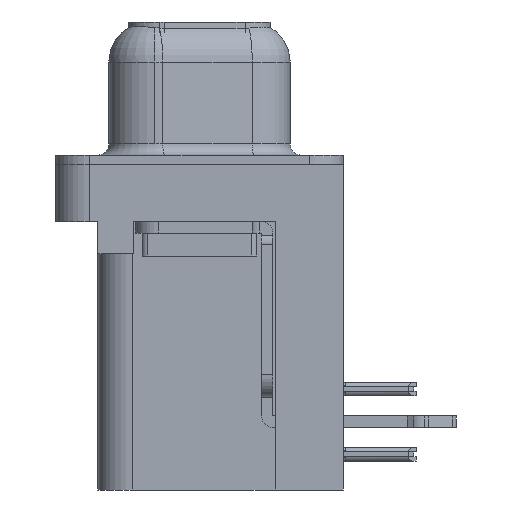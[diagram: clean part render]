
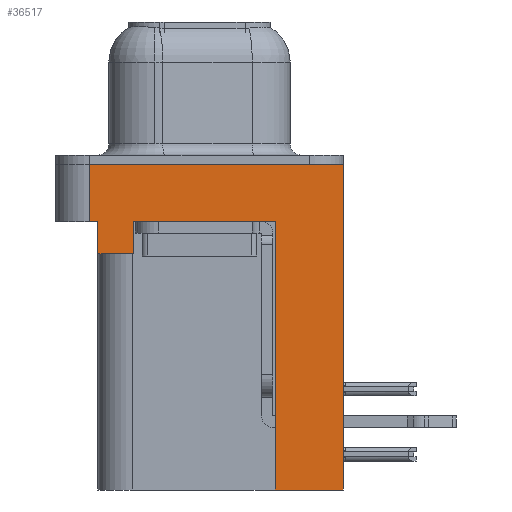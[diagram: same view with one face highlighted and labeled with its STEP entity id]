
A CAD part, left-side view. The second image highlights one B-rep face of the part: STEP entity #36517.
In plain terms, the highlighted planar face has unit normal (-1, 0, 0).
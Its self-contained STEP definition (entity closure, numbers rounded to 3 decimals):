
#898 = DIRECTION ( 'NONE',  ( 0., 0., 1. ) ) ;
#1090 = VERTEX_POINT ( 'NONE', #3404 ) ;
#1162 = CARTESIAN_POINT ( 'NONE',  ( -2.91, 4.425, -2.5 ) ) ;
#2008 = ORIENTED_EDGE ( 'NONE', *, *, #3464, .F. ) ;
#2231 = DIRECTION ( 'NONE',  ( 0., 0., 1. ) ) ;
#2483 = LINE ( 'NONE', #10907, #5870 ) ;
#2527 = LINE ( 'NONE', #36993, #9130 ) ;
#3404 = CARTESIAN_POINT ( 'NONE',  ( -2.91, 4.775, -2.5 ) ) ;
#3464 = EDGE_CURVE ( 'NONE', #19878, #36269, #32067, .T. ) ;
#3587 = EDGE_LOOP ( 'NONE', ( #21074, #10471, #36669, #2008, #30302, #30463, #7401, #21147, #18138, #16201 ) ) ;
#3831 = AXIS2_PLACEMENT_3D ( 'NONE', #22503, #31313, #22687 ) ;
#4296 = EDGE_CURVE ( 'NONE', #1090, #36269, #2483, .T. ) ;
#4725 = LINE ( 'NONE', #10325, #6141 ) ;
#5227 = LINE ( 'NONE', #19285, #10044 ) ;
#5805 = LINE ( 'NONE', #23047, #31759 ) ;
#5870 = VECTOR ( 'NONE', #33771, 1000. ) ;
#6141 = VECTOR ( 'NONE', #13321, 1000. ) ;
#6262 = CARTESIAN_POINT ( 'NONE',  ( -2.91, -6.275, -14.2 ) ) ;
#6846 = VERTEX_POINT ( 'NONE', #6262 ) ;
#7401 = ORIENTED_EDGE ( 'NONE', *, *, #11148, .T. ) ;
#8480 = VERTEX_POINT ( 'NONE', #26962 ) ;
#9016 = DIRECTION ( 'NONE',  ( 0., 0., 1. ) ) ;
#9044 = CARTESIAN_POINT ( 'NONE',  ( -2.91, -3.295, -14.2 ) ) ;
#9060 = DIRECTION ( 'NONE',  ( 0., 1., 0. ) ) ;
#9130 = VECTOR ( 'NONE', #9060, 1000. ) ;
#9145 = CARTESIAN_POINT ( 'NONE',  ( -2.91, 2.895, -3.9 ) ) ;
#9480 = EDGE_CURVE ( 'NONE', #27949, #31424, #14286, .T. ) ;
#9493 = EDGE_CURVE ( 'NONE', #15021, #8480, #26099, .T. ) ;
#9781 = EDGE_CURVE ( 'NONE', #6846, #8480, #5227, .T. ) ;
#10044 = VECTOR ( 'NONE', #2231, 1000. ) ;
#10325 = CARTESIAN_POINT ( 'NONE',  ( -2.91, -6.275, -2.5 ) ) ;
#10471 = ORIENTED_EDGE ( 'NONE', *, *, #26004, .F. ) ;
#10907 = CARTESIAN_POINT ( 'NONE',  ( -2.91, -6.275, -2.5 ) ) ;
#10985 = CARTESIAN_POINT ( 'NONE',  ( -2.91, -3.295, -14.2 ) ) ;
#11148 = EDGE_CURVE ( 'NONE', #25898, #31424, #4725, .T. ) ;
#12255 = CARTESIAN_POINT ( 'NONE',  ( -2.91, 2.895, -3.9 ) ) ;
#12529 = EDGE_CURVE ( 'NONE', #6846, #27949, #36653, .T. ) ;
#12693 = CARTESIAN_POINT ( 'NONE',  ( -2.91, -3.295, -2.5 ) ) ;
#13321 = DIRECTION ( 'NONE',  ( 0., -1., 0. ) ) ;
#14056 = EDGE_CURVE ( 'NONE', #22194, #19878, #2527, .T. ) ;
#14103 = DIRECTION ( 'NONE',  ( 0., 0., 1. ) ) ;
#14286 = LINE ( 'NONE', #9044, #18883 ) ;
#15021 = VERTEX_POINT ( 'NONE', #17429 ) ;
#16201 = ORIENTED_EDGE ( 'NONE', *, *, #9781, .T. ) ;
#16905 = FACE_OUTER_BOUND ( 'NONE', #3587, .T. ) ;
#17429 = CARTESIAN_POINT ( 'NONE',  ( -2.91, 4.775, 0. ) ) ;
#17481 = CARTESIAN_POINT ( 'NONE',  ( -2.91, 4.425, -3.9 ) ) ;
#18138 = ORIENTED_EDGE ( 'NONE', *, *, #12529, .F. ) ;
#18387 = EDGE_CURVE ( 'NONE', #22194, #25898, #29031, .T. ) ;
#18883 = VECTOR ( 'NONE', #14103, 1000. ) ;
#19242 = DIRECTION ( 'NONE',  ( 0., 1., 0. ) ) ;
#19285 = CARTESIAN_POINT ( 'NONE',  ( -2.91, -6.275, -2.5 ) ) ;
#19827 = VECTOR ( 'NONE', #19242, 1000. ) ;
#19878 = VERTEX_POINT ( 'NONE', #34134 ) ;
#20303 = DIRECTION ( 'NONE',  ( 0., -1., 0. ) ) ;
#20777 = DIRECTION ( 'NONE',  ( 0., 0., 1. ) ) ;
#21074 = ORIENTED_EDGE ( 'NONE', *, *, #9493, .F. ) ;
#21147 = ORIENTED_EDGE ( 'NONE', *, *, #9480, .F. ) ;
#22194 = VERTEX_POINT ( 'NONE', #12255 ) ;
#22503 = CARTESIAN_POINT ( 'NONE',  ( -2.91, -6.275, -2.5 ) ) ;
#22687 = DIRECTION ( 'NONE',  ( 0., 0., 1. ) ) ;
#22878 = PLANE ( 'NONE',  #3831 ) ;
#23047 = CARTESIAN_POINT ( 'NONE',  ( -2.91, 4.775, -2.5 ) ) ;
#24317 = VECTOR ( 'NONE', #898, 1000. ) ;
#25898 = VERTEX_POINT ( 'NONE', #28119 ) ;
#26004 = EDGE_CURVE ( 'NONE', #1090, #15021, #5805, .T. ) ;
#26099 = LINE ( 'NONE', #28371, #34203 ) ;
#26962 = CARTESIAN_POINT ( 'NONE',  ( -2.91, -6.275, 0. ) ) ;
#27949 = VERTEX_POINT ( 'NONE', #35029 ) ;
#28119 = CARTESIAN_POINT ( 'NONE',  ( -2.91, 2.895, -2.5 ) ) ;
#28371 = CARTESIAN_POINT ( 'NONE',  ( -2.91, -6.275, 0. ) ) ;
#29031 = LINE ( 'NONE', #9145, #24317 ) ;
#30302 = ORIENTED_EDGE ( 'NONE', *, *, #14056, .F. ) ;
#30463 = ORIENTED_EDGE ( 'NONE', *, *, #18387, .T. ) ;
#31313 = DIRECTION ( 'NONE',  ( -1., 0., 0. ) ) ;
#31424 = VERTEX_POINT ( 'NONE', #12693 ) ;
#31759 = VECTOR ( 'NONE', #20777, 1000. ) ;
#32067 = LINE ( 'NONE', #17481, #36948 ) ;
#33771 = DIRECTION ( 'NONE',  ( 0., -1., 0. ) ) ;
#34134 = CARTESIAN_POINT ( 'NONE',  ( -2.91, 4.425, -3.9 ) ) ;
#34203 = VECTOR ( 'NONE', #20303, 1000. ) ;
#35029 = CARTESIAN_POINT ( 'NONE',  ( -2.91, -3.295, -14.2 ) ) ;
#36269 = VERTEX_POINT ( 'NONE', #1162 ) ;
#36517 = ADVANCED_FACE ( 'NONE', ( #16905 ), #22878, .T. ) ;
#36653 = LINE ( 'NONE', #10985, #19827 ) ;
#36669 = ORIENTED_EDGE ( 'NONE', *, *, #4296, .T. ) ;
#36948 = VECTOR ( 'NONE', #9016, 1000. ) ;
#36993 = CARTESIAN_POINT ( 'NONE',  ( -2.91, 4.425, -3.9 ) ) ;
